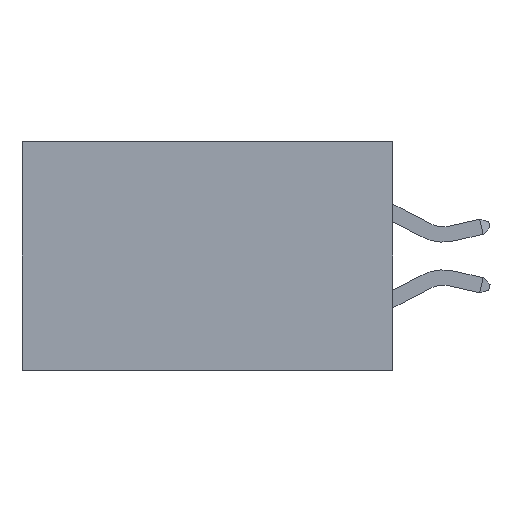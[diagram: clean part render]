
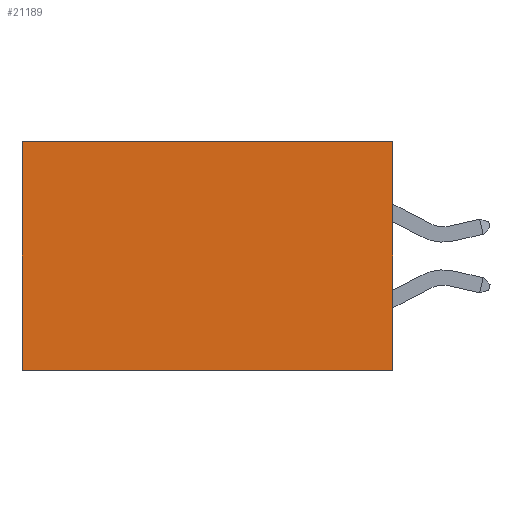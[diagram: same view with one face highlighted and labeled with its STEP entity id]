
A CAD part, left-side view. The second image highlights one B-rep face of the part: STEP entity #21189.
In plain terms, the highlighted planar face has unit normal (-1, 0, 0).
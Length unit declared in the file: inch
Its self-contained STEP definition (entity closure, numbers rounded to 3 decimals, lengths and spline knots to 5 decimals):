
#304 = CARTESIAN_POINT ( 'NONE',  ( 0.2875, 0., -0.37 ) ) ;
#1060 = ORIENTED_EDGE ( 'NONE', *, *, #15551, .T. ) ;
#2293 = ORIENTED_EDGE ( 'NONE', *, *, #10485, .T. ) ;
#2529 = VERTEX_POINT ( 'NONE', #11800 ) ;
#3264 = EDGE_CURVE ( 'NONE', #27142, #30421, #16054, .T. ) ;
#4128 = CARTESIAN_POINT ( 'NONE',  ( 0.2875, 0., 0. ) ) ;
#4732 = VECTOR ( 'NONE', #6846, 39.37008 ) ;
#6529 = CARTESIAN_POINT ( 'NONE',  ( 0.2875, 0., 0. ) ) ;
#6846 = DIRECTION ( 'NONE',  ( 0., 0., -1. ) ) ;
#10262 = DIRECTION ( 'NONE',  ( 0., 1., 0. ) ) ;
#10485 = EDGE_CURVE ( 'NONE', #27142, #2529, #18216, .T. ) ;
#10608 = VECTOR ( 'NONE', #16547, 39.37008 ) ;
#11745 = CARTESIAN_POINT ( 'NONE',  ( 0.2875, 0.6, 0. ) ) ;
#11800 = CARTESIAN_POINT ( 'NONE',  ( 0.2875, 0.6, 0. ) ) ;
#13172 = LINE ( 'NONE', #304, #18999 ) ;
#13384 = VERTEX_POINT ( 'NONE', #17265 ) ;
#14546 = ORIENTED_EDGE ( 'NONE', *, *, #21895, .F. ) ;
#15551 = EDGE_CURVE ( 'NONE', #2529, #13384, #18809, .T. ) ;
#15866 = VECTOR ( 'NONE', #26555, 39.37008 ) ;
#16054 = LINE ( 'NONE', #6529, #4732 ) ;
#16547 = DIRECTION ( 'NONE',  ( 0., 0., -1. ) ) ;
#17265 = CARTESIAN_POINT ( 'NONE',  ( 0.2875, 0.6, -0.37 ) ) ;
#17968 = PLANE ( 'NONE',  #26795 ) ;
#18216 = LINE ( 'NONE', #23635, #15866 ) ;
#18809 = LINE ( 'NONE', #11745, #10608 ) ;
#18999 = VECTOR ( 'NONE', #10262, 39.37008 ) ;
#19332 = ORIENTED_EDGE ( 'NONE', *, *, #3264, .F. ) ;
#21189 = ADVANCED_FACE ( 'NONE', ( #22542 ), #17968, .F. ) ;
#21895 = EDGE_CURVE ( 'NONE', #30421, #13384, #13172, .T. ) ;
#22542 = FACE_OUTER_BOUND ( 'NONE', #24317, .T. ) ;
#23635 = CARTESIAN_POINT ( 'NONE',  ( 0.2875, 0., 0. ) ) ;
#24317 = EDGE_LOOP ( 'NONE', ( #1060, #14546, #19332, #2293 ) ) ;
#25584 = CARTESIAN_POINT ( 'NONE',  ( 0.2875, 0., 0. ) ) ;
#25685 = DIRECTION ( 'NONE',  ( 0., 0., -1. ) ) ;
#26555 = DIRECTION ( 'NONE',  ( 0., 1., 0. ) ) ;
#26795 = AXIS2_PLACEMENT_3D ( 'NONE', #25584, #27846, #25685 ) ;
#27142 = VERTEX_POINT ( 'NONE', #4128 ) ;
#27846 = DIRECTION ( 'NONE',  ( 1., 0., 0. ) ) ;
#28116 = CARTESIAN_POINT ( 'NONE',  ( 0.2875, 0., -0.37 ) ) ;
#30421 = VERTEX_POINT ( 'NONE', #28116 ) ;
